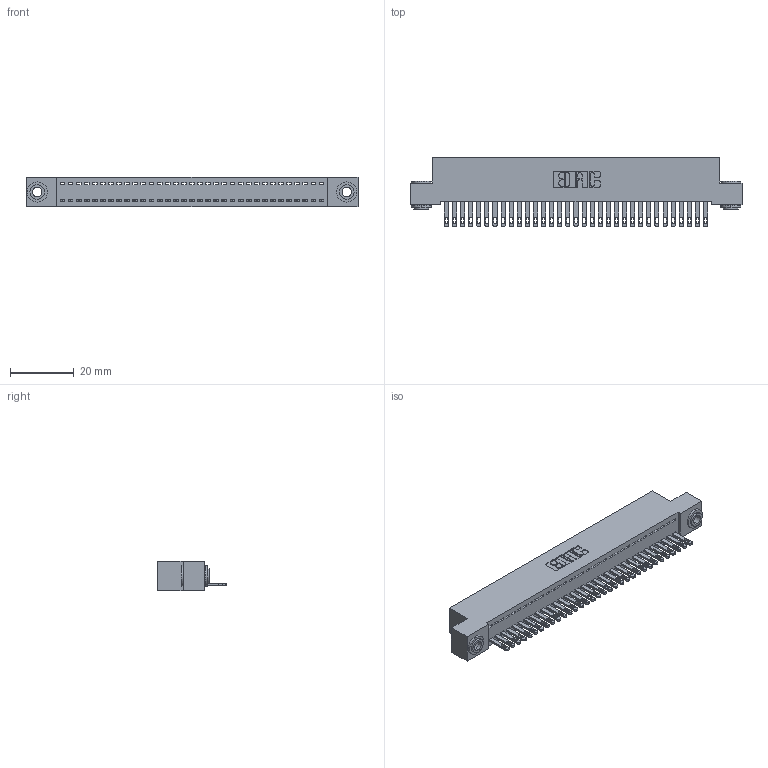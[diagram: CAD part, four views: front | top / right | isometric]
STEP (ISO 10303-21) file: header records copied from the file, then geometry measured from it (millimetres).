
FILE_DESCRIPTION (( 'STEP AP203' ), '1' );
FILE_NAME ('892-033-500-103.STEP', '2020-09-21T15:30:25', ( '' ), ( '' ), 'SwSTEP 2.0', 'SolidWorks 2020', '' );
FILE_SCHEMA (( 'CONFIG_CONTROL_DESIGN' ));
Length unit declared in the file: inch
Products named in the file (4): 342-250-002_345-250-002-102; 892-033-500-103; 345-292-001_345-293-100; 842 Part_.156 TH
Assembly tree (36 placements, depth 2):
  892-033-500-103
    842 Part_.156 TH
    345-292-001_345-293-100  x33
    342-250-002_345-250-002-102  x2
Bounding box: 104.14 x 21.85 x 9.4 mm (x, y, z)
Volume: 9141.1 mm3; surface area: 13546.4 mm2
Topology: 36 solids, 36 shells, 1930 faces, 5919 edges, 3942 vertices
Faces by surface type: plane 1264, cylinder 658, cone 8
Entity records: 21786 total; most frequent: CARTESIAN_POINT 3736, ORIENTED_EDGE 3698, DIRECTION 3205, EDGE_CURVE 1849, LINE 1693, VECTOR 1693, VERTEX_POINT 1230, AXIS2_PLACEMENT_3D 756
